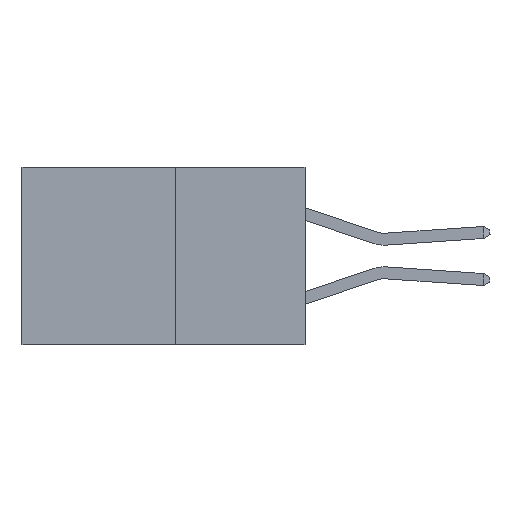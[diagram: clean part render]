
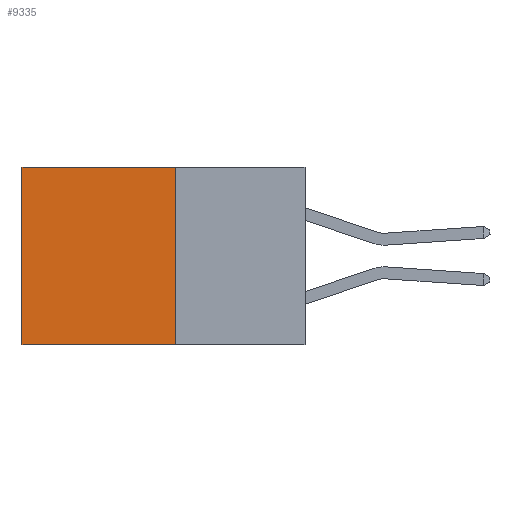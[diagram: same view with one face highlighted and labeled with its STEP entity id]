
A CAD part, left-side view. The second image highlights one B-rep face of the part: STEP entity #9335.
In plain terms, the highlighted planar face has unit normal (-1, 0, 0).
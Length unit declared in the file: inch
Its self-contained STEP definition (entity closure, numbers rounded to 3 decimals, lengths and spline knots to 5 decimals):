
#122 = CARTESIAN_POINT ( 'NONE',  ( 0.277, 0.59, -0.37 ) ) ;
#864 = DIRECTION ( 'NONE',  ( 0., 0., -1. ) ) ;
#1552 = CARTESIAN_POINT ( 'NONE',  ( 0.277, 0.59, 0. ) ) ;
#2710 = VERTEX_POINT ( 'NONE', #12471 ) ;
#2769 = LINE ( 'NONE', #6590, #12840 ) ;
#2859 = EDGE_LOOP ( 'NONE', ( #11584, #15688, #13399, #10888 ) ) ;
#3797 = EDGE_CURVE ( 'NONE', #11204, #7956, #8818, .T. ) ;
#4063 = LINE ( 'NONE', #5019, #10615 ) ;
#4306 = CARTESIAN_POINT ( 'NONE',  ( 0.277, 0.27, 0. ) ) ;
#4491 = DIRECTION ( 'NONE',  ( 0., 1., 0. ) ) ;
#5019 = CARTESIAN_POINT ( 'NONE',  ( 0.277, 0.27, -0.37 ) ) ;
#5393 = PLANE ( 'NONE',  #9965 ) ;
#5419 = EDGE_CURVE ( 'NONE', #7956, #5427, #2769, .T. ) ;
#5427 = VERTEX_POINT ( 'NONE', #122 ) ;
#5583 = VECTOR ( 'NONE', #864, 39.37008 ) ;
#6590 = CARTESIAN_POINT ( 'NONE',  ( 0.277, 0.59, -0.37 ) ) ;
#6723 = DIRECTION ( 'NONE',  ( 1., 0., 0. ) ) ;
#7401 = CARTESIAN_POINT ( 'NONE',  ( 0.277, 0.27, -0.37 ) ) ;
#7956 = VERTEX_POINT ( 'NONE', #1552 ) ;
#8342 = CARTESIAN_POINT ( 'NONE',  ( 0.277, 0.27, 0. ) ) ;
#8818 = LINE ( 'NONE', #4306, #11862 ) ;
#8820 = FACE_OUTER_BOUND ( 'NONE', #2859, .T. ) ;
#9100 = LINE ( 'NONE', #7401, #5583 ) ;
#9335 = ADVANCED_FACE ( 'NONE', ( #8820 ), #5393, .F. ) ;
#9965 = AXIS2_PLACEMENT_3D ( 'NONE', #13270, #6723, #15851 ) ;
#10615 = VECTOR ( 'NONE', #15495, 39.37008 ) ;
#10888 = ORIENTED_EDGE ( 'NONE', *, *, #3797, .T. ) ;
#11204 = VERTEX_POINT ( 'NONE', #8342 ) ;
#11584 = ORIENTED_EDGE ( 'NONE', *, *, #5419, .T. ) ;
#11862 = VECTOR ( 'NONE', #4491, 39.37008 ) ;
#12471 = CARTESIAN_POINT ( 'NONE',  ( 0.277, 0.27, -0.37 ) ) ;
#12840 = VECTOR ( 'NONE', #14484, 39.37008 ) ;
#12849 = EDGE_CURVE ( 'NONE', #2710, #5427, #4063, .T. ) ;
#13270 = CARTESIAN_POINT ( 'NONE',  ( 0.277, 0.27, -0.37 ) ) ;
#13399 = ORIENTED_EDGE ( 'NONE', *, *, #15911, .F. ) ;
#14484 = DIRECTION ( 'NONE',  ( 0., 0., -1. ) ) ;
#15495 = DIRECTION ( 'NONE',  ( 0., 1., 0. ) ) ;
#15688 = ORIENTED_EDGE ( 'NONE', *, *, #12849, .F. ) ;
#15851 = DIRECTION ( 'NONE',  ( 0., 0., -1. ) ) ;
#15911 = EDGE_CURVE ( 'NONE', #11204, #2710, #9100, .T. ) ;
